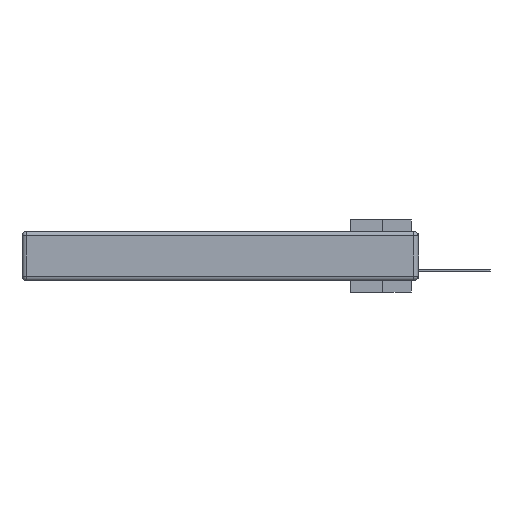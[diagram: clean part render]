
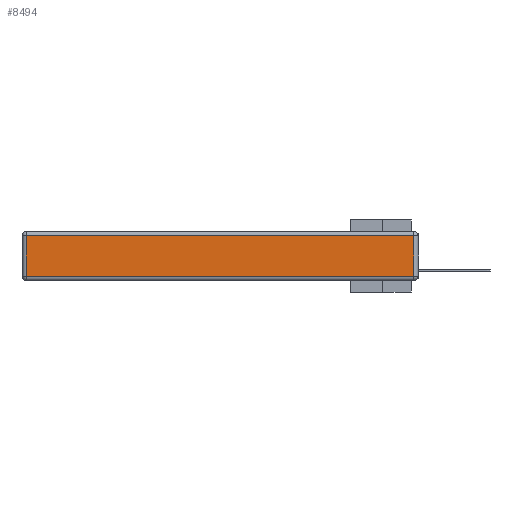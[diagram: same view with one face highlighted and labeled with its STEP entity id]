
A CAD part, left-side view. The second image highlights one B-rep face of the part: STEP entity #8494.
In plain terms, the highlighted planar face has unit normal (-1, 0, 0).
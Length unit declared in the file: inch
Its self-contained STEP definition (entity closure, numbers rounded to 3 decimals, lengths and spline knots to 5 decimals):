
#568 = EDGE_CURVE ( 'NONE', #9945, #13449, #3627, .T. ) ;
#1192 = VECTOR ( 'NONE', #36457, 39.37008 ) ;
#2548 = CARTESIAN_POINT ( 'NONE',  ( 0., 2.72, -0.03 ) ) ;
#2750 = DIRECTION ( 'NONE',  ( 0., 0., 1. ) ) ;
#2868 = DIRECTION ( 'NONE',  ( -1., 0., 0. ) ) ;
#3398 = ORIENTED_EDGE ( 'NONE', *, *, #568, .T. ) ;
#3627 = LINE ( 'NONE', #9140, #11298 ) ;
#7537 = CARTESIAN_POINT ( 'NONE',  ( 0., 0.03, -0.343 ) ) ;
#8200 = PLANE ( 'NONE',  #32450 ) ;
#8385 = CARTESIAN_POINT ( 'NONE',  ( 0., 0., -0.343 ) ) ;
#8494 = ADVANCED_FACE ( 'NONE', ( #27680 ), #8200, .T. ) ;
#8556 = VECTOR ( 'NONE', #32063, 39.37008 ) ;
#9140 = CARTESIAN_POINT ( 'NONE',  ( 0., 0., -0.313 ) ) ;
#9945 = VERTEX_POINT ( 'NONE', #19738 ) ;
#11298 = VECTOR ( 'NONE', #29338, 39.37008 ) ;
#11304 = LINE ( 'NONE', #28163, #1192 ) ;
#11866 = CARTESIAN_POINT ( 'NONE',  ( 0., 0.03, -0.313 ) ) ;
#13449 = VERTEX_POINT ( 'NONE', #11866 ) ;
#14095 = EDGE_CURVE ( 'NONE', #13449, #15279, #16791, .T. ) ;
#15064 = VECTOR ( 'NONE', #2750, 39.37008 ) ;
#15279 = VERTEX_POINT ( 'NONE', #20279 ) ;
#16791 = LINE ( 'NONE', #7537, #15064 ) ;
#18876 = EDGE_LOOP ( 'NONE', ( #3398, #34224, #28376, #26872 ) ) ;
#19738 = CARTESIAN_POINT ( 'NONE',  ( 0., 2.72, -0.313 ) ) ;
#20279 = CARTESIAN_POINT ( 'NONE',  ( 0., 0.03, -0.03 ) ) ;
#20390 = LINE ( 'NONE', #26151, #8556 ) ;
#20493 = EDGE_CURVE ( 'NONE', #15279, #22632, #11304, .T. ) ;
#22632 = VERTEX_POINT ( 'NONE', #2548 ) ;
#26151 = CARTESIAN_POINT ( 'NONE',  ( 0., 2.72, -0.343 ) ) ;
#26872 = ORIENTED_EDGE ( 'NONE', *, *, #32548, .T. ) ;
#27680 = FACE_OUTER_BOUND ( 'NONE', #18876, .T. ) ;
#28163 = CARTESIAN_POINT ( 'NONE',  ( 0., 2.75, -0.03 ) ) ;
#28376 = ORIENTED_EDGE ( 'NONE', *, *, #20493, .T. ) ;
#29338 = DIRECTION ( 'NONE',  ( 0., -1., 0. ) ) ;
#30637 = DIRECTION ( 'NONE',  ( 0., 0., 1. ) ) ;
#32063 = DIRECTION ( 'NONE',  ( 0., 0., -1. ) ) ;
#32450 = AXIS2_PLACEMENT_3D ( 'NONE', #8385, #2868, #30637 ) ;
#32548 = EDGE_CURVE ( 'NONE', #22632, #9945, #20390, .T. ) ;
#34224 = ORIENTED_EDGE ( 'NONE', *, *, #14095, .T. ) ;
#36457 = DIRECTION ( 'NONE',  ( 0., 1., 0. ) ) ;
